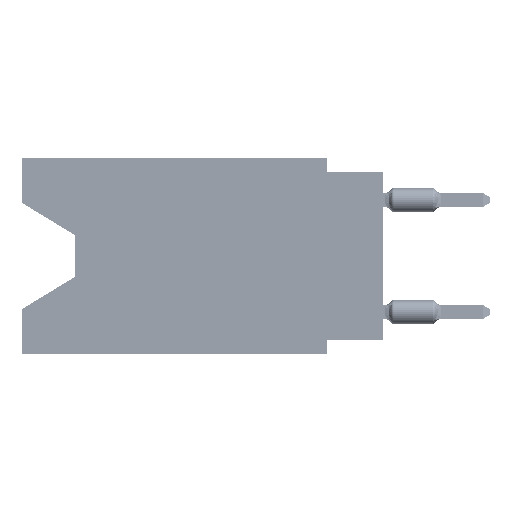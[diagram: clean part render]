
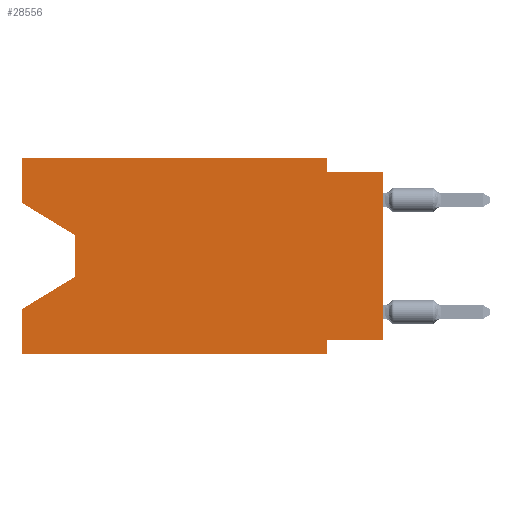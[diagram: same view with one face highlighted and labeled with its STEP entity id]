
A CAD part, left-side view. The second image highlights one B-rep face of the part: STEP entity #28556.
In plain terms, the highlighted planar face has unit normal (-1, 0, 0).
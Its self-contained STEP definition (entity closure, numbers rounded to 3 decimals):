
#162 = LINE ( 'NONE', #61587, #23639 ) ;
#692 = EDGE_LOOP ( 'NONE', ( #66233, #39543, #54022, #15422, #26176, #25086, #1693, #35956, #28062, #18469, #21490, #35265 ) ) ;
#1533 = EDGE_CURVE ( 'NONE', #12482, #59619, #5524, .T. ) ;
#1665 = AXIS2_PLACEMENT_3D ( 'NONE', #4421, #60735, #15762 ) ;
#1693 = ORIENTED_EDGE ( 'NONE', *, *, #7756, .F. ) ;
#1943 = LINE ( 'NONE', #51713, #63775 ) ;
#2638 = LINE ( 'NONE', #24959, #45012 ) ;
#3341 = DIRECTION ( 'NONE',  ( 0., 0., -1. ) ) ;
#3914 = DIRECTION ( 'NONE',  ( 0., 0., -1. ) ) ;
#4421 = CARTESIAN_POINT ( 'NONE',  ( 0., 16.383, 0. ) ) ;
#5524 = LINE ( 'NONE', #45387, #43476 ) ;
#6127 = EDGE_CURVE ( 'NONE', #43804, #48588, #30413, .T. ) ;
#6503 = VECTOR ( 'NONE', #17847, 1000. ) ;
#6993 = DIRECTION ( 'NONE',  ( 0., -0.855, -0.519 ) ) ;
#7756 = EDGE_CURVE ( 'NONE', #71612, #21591, #67918, .T. ) ;
#8667 = DIRECTION ( 'NONE',  ( 0., 0., 1. ) ) ;
#9250 = DIRECTION ( 'NONE',  ( 0., -1., 0. ) ) ;
#10709 = VERTEX_POINT ( 'NONE', #57477 ) ;
#12482 = VERTEX_POINT ( 'NONE', #54100 ) ;
#12759 = VECTOR ( 'NONE', #18039, 1000. ) ;
#12915 = LINE ( 'NONE', #41081, #46179 ) ;
#15422 = ORIENTED_EDGE ( 'NONE', *, *, #52024, .F. ) ;
#15762 = DIRECTION ( 'NONE',  ( 0., 0., -1. ) ) ;
#16980 = DIRECTION ( 'NONE',  ( 0., 0., 1. ) ) ;
#17159 = VERTEX_POINT ( 'NONE', #37456 ) ;
#17847 = DIRECTION ( 'NONE',  ( 0., 1., 0. ) ) ;
#18039 = DIRECTION ( 'NONE',  ( 0., 0.855, -0.519 ) ) ;
#18469 = ORIENTED_EDGE ( 'NONE', *, *, #59746, .F. ) ;
#18567 = CARTESIAN_POINT ( 'NONE',  ( 0., 0., 0. ) ) ;
#21110 = CARTESIAN_POINT ( 'NONE',  ( 0., 13.97, -3.505 ) ) ;
#21490 = ORIENTED_EDGE ( 'NONE', *, *, #1533, .F. ) ;
#21591 = VERTEX_POINT ( 'NONE', #24221 ) ;
#22547 = LINE ( 'NONE', #33509, #58402 ) ;
#23118 = CARTESIAN_POINT ( 'NONE',  ( 0., 13.97, -3.505 ) ) ;
#23627 = DIRECTION ( 'NONE',  ( 0., 0., 1. ) ) ;
#23639 = VECTOR ( 'NONE', #16980, 1000. ) ;
#24221 = CARTESIAN_POINT ( 'NONE',  ( 0., 2.54, -8.255 ) ) ;
#24959 = CARTESIAN_POINT ( 'NONE',  ( 0., 2.54, -8.89 ) ) ;
#25086 = ORIENTED_EDGE ( 'NONE', *, *, #29723, .F. ) ;
#25818 = CARTESIAN_POINT ( 'NONE',  ( 0., 2.54, -0.635 ) ) ;
#26176 = ORIENTED_EDGE ( 'NONE', *, *, #59955, .T. ) ;
#28062 = ORIENTED_EDGE ( 'NONE', *, *, #58513, .F. ) ;
#28556 = ADVANCED_FACE ( 'NONE', ( #65853 ), #32233, .F. ) ;
#29083 = VECTOR ( 'NONE', #8667, 1000. ) ;
#29723 = EDGE_CURVE ( 'NONE', #21591, #10709, #2638, .T. ) ;
#30413 = LINE ( 'NONE', #41378, #60262 ) ;
#31721 = LINE ( 'NONE', #21110, #59872 ) ;
#32233 = PLANE ( 'NONE',  #1665 ) ;
#33344 = CARTESIAN_POINT ( 'NONE',  ( 0., 16.383, -6.852 ) ) ;
#33509 = CARTESIAN_POINT ( 'NONE',  ( 0., 16.383, 0. ) ) ;
#34303 = CARTESIAN_POINT ( 'NONE',  ( 0., 0., -8.255 ) ) ;
#35265 = ORIENTED_EDGE ( 'NONE', *, *, #36918, .F. ) ;
#35956 = ORIENTED_EDGE ( 'NONE', *, *, #50549, .T. ) ;
#35962 = DIRECTION ( 'NONE',  ( 0., 0., -1. ) ) ;
#36918 = EDGE_CURVE ( 'NONE', #43804, #12482, #162, .T. ) ;
#37040 = LINE ( 'NONE', #64827, #57968 ) ;
#37456 = CARTESIAN_POINT ( 'NONE',  ( 0., 16.383, -8.89 ) ) ;
#39143 = EDGE_CURVE ( 'NONE', #48588, #43988, #31721, .T. ) ;
#39543 = ORIENTED_EDGE ( 'NONE', *, *, #39143, .T. ) ;
#40958 = EDGE_CURVE ( 'NONE', #43988, #41175, #47653, .T. ) ;
#41012 = VERTEX_POINT ( 'NONE', #59696 ) ;
#41081 = CARTESIAN_POINT ( 'NONE',  ( 0., 0., -0.635 ) ) ;
#41175 = VERTEX_POINT ( 'NONE', #33344 ) ;
#41378 = CARTESIAN_POINT ( 'NONE',  ( 0., 16.383, -2.038 ) ) ;
#41800 = VERTEX_POINT ( 'NONE', #25818 ) ;
#43476 = VECTOR ( 'NONE', #55634, 1000. ) ;
#43804 = VERTEX_POINT ( 'NONE', #59537 ) ;
#43988 = VERTEX_POINT ( 'NONE', #60630 ) ;
#45012 = VECTOR ( 'NONE', #3341, 1000. ) ;
#45387 = CARTESIAN_POINT ( 'NONE',  ( 0., 16.383, 0. ) ) ;
#46179 = VECTOR ( 'NONE', #63731, 1000. ) ;
#47653 = LINE ( 'NONE', #64093, #12759 ) ;
#48588 = VERTEX_POINT ( 'NONE', #23118 ) ;
#50549 = EDGE_CURVE ( 'NONE', #71612, #41012, #58767, .T. ) ;
#50872 = CARTESIAN_POINT ( 'NONE',  ( 0., 0., -8.255 ) ) ;
#51713 = CARTESIAN_POINT ( 'NONE',  ( 0., 2.54, 0. ) ) ;
#52024 = EDGE_CURVE ( 'NONE', #17159, #41175, #22547, .T. ) ;
#54022 = ORIENTED_EDGE ( 'NONE', *, *, #40958, .T. ) ;
#54100 = CARTESIAN_POINT ( 'NONE',  ( 0., 16.383, 0. ) ) ;
#55634 = DIRECTION ( 'NONE',  ( 0., -1., 0. ) ) ;
#57477 = CARTESIAN_POINT ( 'NONE',  ( 0., 2.54, -8.89 ) ) ;
#57968 = VECTOR ( 'NONE', #9250, 1000. ) ;
#58402 = VECTOR ( 'NONE', #23627, 1000. ) ;
#58513 = EDGE_CURVE ( 'NONE', #41800, #41012, #12915, .T. ) ;
#58767 = LINE ( 'NONE', #18567, #29083 ) ;
#59537 = CARTESIAN_POINT ( 'NONE',  ( 0., 16.383, -2.038 ) ) ;
#59619 = VERTEX_POINT ( 'NONE', #61590 ) ;
#59696 = CARTESIAN_POINT ( 'NONE',  ( 0., 0., -0.635 ) ) ;
#59746 = EDGE_CURVE ( 'NONE', #59619, #41800, #1943, .T. ) ;
#59872 = VECTOR ( 'NONE', #3914, 1000. ) ;
#59955 = EDGE_CURVE ( 'NONE', #17159, #10709, #37040, .T. ) ;
#60262 = VECTOR ( 'NONE', #6993, 1000. ) ;
#60630 = CARTESIAN_POINT ( 'NONE',  ( 0., 13.97, -5.385 ) ) ;
#60735 = DIRECTION ( 'NONE',  ( 1., 0., 0. ) ) ;
#61587 = CARTESIAN_POINT ( 'NONE',  ( 0., 16.383, 0. ) ) ;
#61590 = CARTESIAN_POINT ( 'NONE',  ( 0., 2.54, 0. ) ) ;
#63731 = DIRECTION ( 'NONE',  ( 0., -1., 0. ) ) ;
#63775 = VECTOR ( 'NONE', #35962, 1000. ) ;
#64093 = CARTESIAN_POINT ( 'NONE',  ( 0., 13.97, -5.385 ) ) ;
#64827 = CARTESIAN_POINT ( 'NONE',  ( 0., 16.383, -8.89 ) ) ;
#65853 = FACE_OUTER_BOUND ( 'NONE', #692, .T. ) ;
#66233 = ORIENTED_EDGE ( 'NONE', *, *, #6127, .T. ) ;
#67918 = LINE ( 'NONE', #34303, #6503 ) ;
#71612 = VERTEX_POINT ( 'NONE', #50872 ) ;
